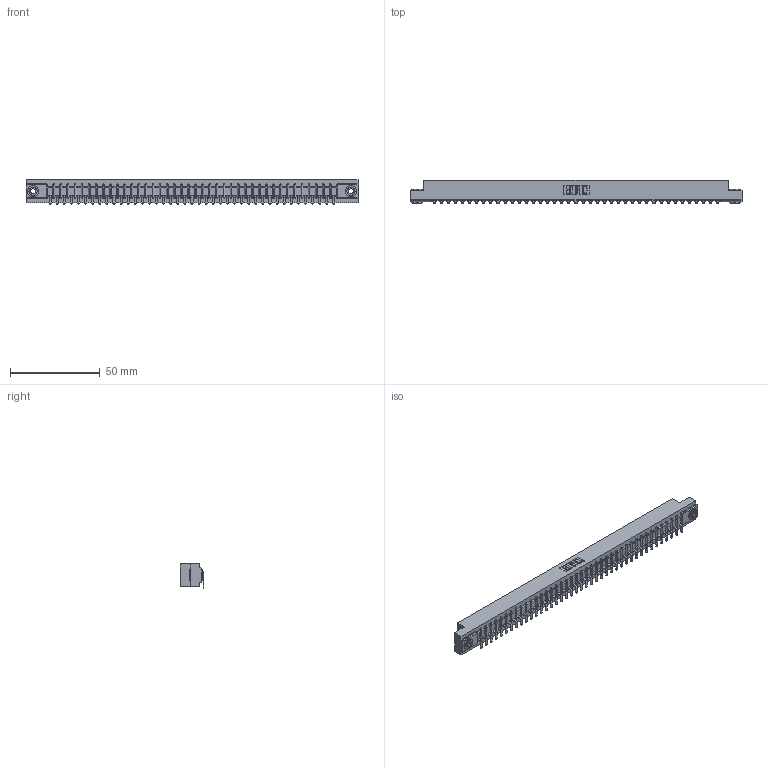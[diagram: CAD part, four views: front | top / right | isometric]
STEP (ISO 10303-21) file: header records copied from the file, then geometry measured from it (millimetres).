
FILE_DESCRIPTION (( 'STEP AP203' ), '1' );
FILE_NAME ('357-041-453-103.STEP', '2020-10-03T08:42:13', ( '' ), ( '' ), 'SwSTEP 2.0', 'SolidWorks 2020', '' );
FILE_SCHEMA (( 'CONFIG_CONTROL_DESIGN' ));
Length unit declared in the file: inch
Products named in the file (4): 357-041-453-103; 307 Part_.156 Dia Mounting Holes; 307-290-002_553; 345-250-002_345-250-002-102
Assembly tree (44 placements, depth 2):
  357-041-453-103
    307 Part_.156 Dia Mounting Holes
    307-290-002_553  x41
    345-250-002_345-250-002-102  x2
Bounding box: 185.47 x 13.36 x 13.5 mm (x, y, z)
Volume: 19841.4 mm3; surface area: 25168.2 mm2
Topology: 44 solids, 44 shells, 3410 faces, 10439 edges, 6842 vertices
Faces by surface type: plane 2021, cylinder 1297, sphere 84, cone 8
Entity records: 37191 total; most frequent: CARTESIAN_POINT 6253, ORIENTED_EDGE 6234, DIRECTION 6091, EDGE_CURVE 3117, LINE 2379, VECTOR 2379, VERTEX_POINT 2018, AXIS2_PLACEMENT_3D 1856
